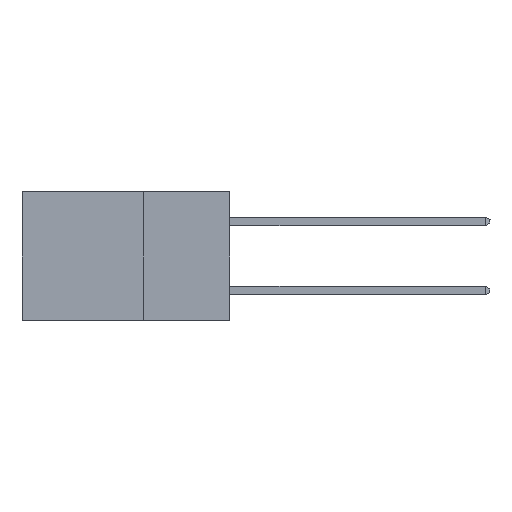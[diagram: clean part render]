
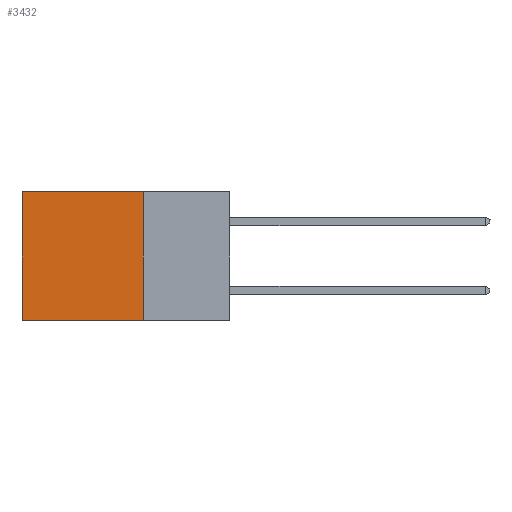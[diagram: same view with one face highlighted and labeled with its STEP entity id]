
A CAD part, left-side view. The second image highlights one B-rep face of the part: STEP entity #3432.
In plain terms, the highlighted planar face has unit normal (-1, 0, 0).
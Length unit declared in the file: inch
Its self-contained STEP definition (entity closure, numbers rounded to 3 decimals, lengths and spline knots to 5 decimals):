
#75 = CARTESIAN_POINT ( 'NONE',  ( 0.2615, 0.6, -0.37 ) ) ;
#636 = ORIENTED_EDGE ( 'NONE', *, *, #5242, .F. ) ;
#902 = ORIENTED_EDGE ( 'NONE', *, *, #8059, .T. ) ;
#909 = CARTESIAN_POINT ( 'NONE',  ( 0.2615, 0.6, 0. ) ) ;
#1094 = LINE ( 'NONE', #9784, #5402 ) ;
#1629 = LINE ( 'NONE', #8711, #4446 ) ;
#1727 = VERTEX_POINT ( 'NONE', #4071 ) ;
#2545 = ORIENTED_EDGE ( 'NONE', *, *, #8955, .T. ) ;
#2699 = CARTESIAN_POINT ( 'NONE',  ( 0.2615, 0.25, -0.37 ) ) ;
#3043 = AXIS2_PLACEMENT_3D ( 'NONE', #2699, #9538, #12471 ) ;
#3220 = CARTESIAN_POINT ( 'NONE',  ( 0.2615, 0.25, -0.37 ) ) ;
#3432 = ADVANCED_FACE ( 'NONE', ( #8598 ), #4560, .F. ) ;
#3781 = VECTOR ( 'NONE', #4818, 39.37008 ) ;
#4071 = CARTESIAN_POINT ( 'NONE',  ( 0.2615, 0.6, -0.37 ) ) ;
#4249 = EDGE_LOOP ( 'NONE', ( #2545, #11917, #636, #902 ) ) ;
#4446 = VECTOR ( 'NONE', #10241, 39.37008 ) ;
#4560 = PLANE ( 'NONE',  #3043 ) ;
#4643 = CARTESIAN_POINT ( 'NONE',  ( 0.2615, 0.25, 0. ) ) ;
#4807 = VERTEX_POINT ( 'NONE', #4643 ) ;
#4818 = DIRECTION ( 'NONE',  ( 0., 0., -1. ) ) ;
#5242 = EDGE_CURVE ( 'NONE', #4807, #10443, #1629, .T. ) ;
#5402 = VECTOR ( 'NONE', #7688, 39.37008 ) ;
#5774 = LINE ( 'NONE', #75, #3781 ) ;
#7631 = VERTEX_POINT ( 'NONE', #909 ) ;
#7688 = DIRECTION ( 'NONE',  ( 0., 1., 0. ) ) ;
#7928 = CARTESIAN_POINT ( 'NONE',  ( 0.2615, 0.25, 0. ) ) ;
#8059 = EDGE_CURVE ( 'NONE', #4807, #7631, #8821, .T. ) ;
#8598 = FACE_OUTER_BOUND ( 'NONE', #4249, .T. ) ;
#8711 = CARTESIAN_POINT ( 'NONE',  ( 0.2615, 0.25, -0.37 ) ) ;
#8821 = LINE ( 'NONE', #7928, #9078 ) ;
#8955 = EDGE_CURVE ( 'NONE', #7631, #1727, #5774, .T. ) ;
#9078 = VECTOR ( 'NONE', #9764, 39.37008 ) ;
#9455 = EDGE_CURVE ( 'NONE', #10443, #1727, #1094, .T. ) ;
#9538 = DIRECTION ( 'NONE',  ( 1., 0., 0. ) ) ;
#9764 = DIRECTION ( 'NONE',  ( 0., 1., 0. ) ) ;
#9784 = CARTESIAN_POINT ( 'NONE',  ( 0.2615, 0.25, -0.37 ) ) ;
#10241 = DIRECTION ( 'NONE',  ( 0., 0., -1. ) ) ;
#10443 = VERTEX_POINT ( 'NONE', #3220 ) ;
#11917 = ORIENTED_EDGE ( 'NONE', *, *, #9455, .F. ) ;
#12471 = DIRECTION ( 'NONE',  ( 0., 0., -1. ) ) ;
